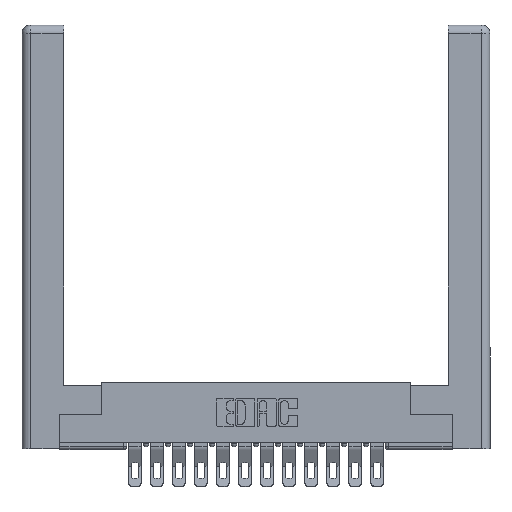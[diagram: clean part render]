
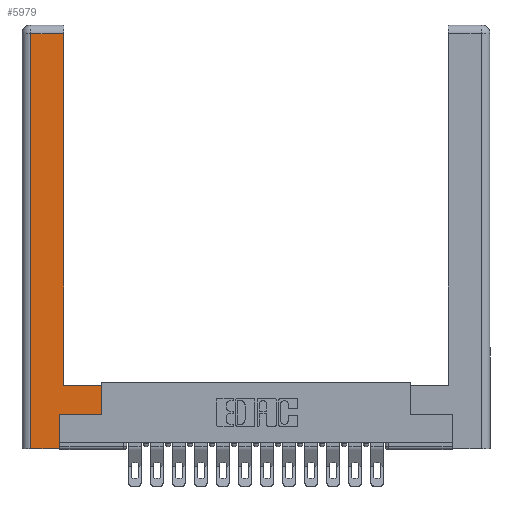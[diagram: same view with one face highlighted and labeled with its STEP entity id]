
A CAD part, top view. The second image highlights one B-rep face of the part: STEP entity #5979.
In plain terms, the highlighted planar face has unit normal (0, 0, 1).
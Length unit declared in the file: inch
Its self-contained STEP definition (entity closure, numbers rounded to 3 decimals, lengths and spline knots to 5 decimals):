
#29 = EDGE_CURVE ( 'NONE', #13177, #4163, #8452, .T. ) ;
#138 = DIRECTION ( 'NONE',  ( 0., 1., 0. ) ) ;
#176 = DIRECTION ( 'NONE',  ( -1., 0., 0. ) ) ;
#444 = VECTOR ( 'NONE', #13873, 39.37008 ) ;
#519 = EDGE_CURVE ( 'NONE', #12789, #6782, #13587, .T. ) ;
#701 = VECTOR ( 'NONE', #12351, 39.37008 ) ;
#1401 = FACE_OUTER_BOUND ( 'NONE', #16584, .T. ) ;
#1549 = CARTESIAN_POINT ( 'NONE',  ( 0.265, 0., 0. ) ) ;
#1747 = CARTESIAN_POINT ( 'NONE',  ( 0.265, 0.245, 0. ) ) ;
#1929 = LINE ( 'NONE', #11272, #3780 ) ;
#2464 = CARTESIAN_POINT ( 'NONE',  ( 0.295, 0.45, 0. ) ) ;
#2493 = DIRECTION ( 'NONE',  ( 0., -1., 0. ) ) ;
#2853 = CARTESIAN_POINT ( 'NONE',  ( 0.0615, 2.94, 0. ) ) ;
#3780 = VECTOR ( 'NONE', #4434, 39.37008 ) ;
#3820 = CARTESIAN_POINT ( 'NONE',  ( 0.565, 0.45, 0. ) ) ;
#3961 = VECTOR ( 'NONE', #12101, 39.37008 ) ;
#4163 = VERTEX_POINT ( 'NONE', #5541 ) ;
#4272 = VECTOR ( 'NONE', #4676, 39.37008 ) ;
#4434 = DIRECTION ( 'NONE',  ( -1., 0., 0. ) ) ;
#4584 = ORIENTED_EDGE ( 'NONE', *, *, #16462, .T. ) ;
#4676 = DIRECTION ( 'NONE',  ( 1., 0., 0. ) ) ;
#5441 = ORIENTED_EDGE ( 'NONE', *, *, #12582, .T. ) ;
#5541 = CARTESIAN_POINT ( 'NONE',  ( 0.0615, 2.94, 0. ) ) ;
#5788 = EDGE_CURVE ( 'NONE', #11200, #13177, #11481, .T. ) ;
#5979 = ADVANCED_FACE ( 'NONE', ( #1401 ), #9511, .F. ) ;
#6210 = EDGE_CURVE ( 'NONE', #6528, #11200, #1929, .T. ) ;
#6473 = CARTESIAN_POINT ( 'NONE',  ( 0.0615, 0., 0. ) ) ;
#6523 = CARTESIAN_POINT ( 'NONE',  ( 0.265, 0.245, 0. ) ) ;
#6528 = VERTEX_POINT ( 'NONE', #16176 ) ;
#6782 = VERTEX_POINT ( 'NONE', #12774 ) ;
#6878 = CARTESIAN_POINT ( 'NONE',  ( 0.295, 3., 0. ) ) ;
#6936 = CARTESIAN_POINT ( 'NONE',  ( 0.295, 2.94, 0. ) ) ;
#7162 = LINE ( 'NONE', #1747, #10782 ) ;
#7522 = CARTESIAN_POINT ( 'NONE',  ( 0.265, 0., 0. ) ) ;
#8015 = EDGE_CURVE ( 'NONE', #17102, #12789, #7162, .T. ) ;
#8407 = ORIENTED_EDGE ( 'NONE', *, *, #5788, .T. ) ;
#8428 = ORIENTED_EDGE ( 'NONE', *, *, #11941, .T. ) ;
#8452 = LINE ( 'NONE', #2853, #444 ) ;
#8682 = DIRECTION ( 'NONE',  ( 0., 1., 0. ) ) ;
#8951 = LINE ( 'NONE', #7522, #4272 ) ;
#9332 = CARTESIAN_POINT ( 'NONE',  ( 0., 0., 0. ) ) ;
#9511 = PLANE ( 'NONE',  #16552 ) ;
#10338 = ORIENTED_EDGE ( 'NONE', *, *, #519, .T. ) ;
#10455 = ORIENTED_EDGE ( 'NONE', *, *, #29, .T. ) ;
#10782 = VECTOR ( 'NONE', #8682, 39.37008 ) ;
#11115 = ORIENTED_EDGE ( 'NONE', *, *, #8015, .T. ) ;
#11200 = VERTEX_POINT ( 'NONE', #2464 ) ;
#11272 = CARTESIAN_POINT ( 'NONE',  ( 0.295, 0.45, 0. ) ) ;
#11481 = LINE ( 'NONE', #6878, #14265 ) ;
#11833 = LINE ( 'NONE', #6473, #13531 ) ;
#11941 = EDGE_CURVE ( 'NONE', #6782, #6528, #13505, .T. ) ;
#12101 = DIRECTION ( 'NONE',  ( 0., 1., 0. ) ) ;
#12351 = DIRECTION ( 'NONE',  ( 1., 0., 0. ) ) ;
#12582 = EDGE_CURVE ( 'NONE', #16927, #17102, #8951, .T. ) ;
#12774 = CARTESIAN_POINT ( 'NONE',  ( 0.565, 0.245, 0. ) ) ;
#12789 = VERTEX_POINT ( 'NONE', #6523 ) ;
#13177 = VERTEX_POINT ( 'NONE', #6936 ) ;
#13505 = LINE ( 'NONE', #3820, #3961 ) ;
#13531 = VECTOR ( 'NONE', #2493, 39.37008 ) ;
#13587 = LINE ( 'NONE', #13852, #701 ) ;
#13852 = CARTESIAN_POINT ( 'NONE',  ( 0.565, 0.245, 0. ) ) ;
#13873 = DIRECTION ( 'NONE',  ( -1., 0., 0. ) ) ;
#14265 = VECTOR ( 'NONE', #138, 39.37008 ) ;
#15539 = ORIENTED_EDGE ( 'NONE', *, *, #6210, .T. ) ;
#16176 = CARTESIAN_POINT ( 'NONE',  ( 0.565, 0.45, 0. ) ) ;
#16341 = CARTESIAN_POINT ( 'NONE',  ( 0.0615, 0., 0. ) ) ;
#16462 = EDGE_CURVE ( 'NONE', #4163, #16927, #11833, .T. ) ;
#16552 = AXIS2_PLACEMENT_3D ( 'NONE', #9332, #17513, #176 ) ;
#16584 = EDGE_LOOP ( 'NONE', ( #8407, #10455, #4584, #5441, #11115, #10338, #8428, #15539 ) ) ;
#16927 = VERTEX_POINT ( 'NONE', #16341 ) ;
#17102 = VERTEX_POINT ( 'NONE', #1549 ) ;
#17513 = DIRECTION ( 'NONE',  ( 0., 0., -1. ) ) ;
